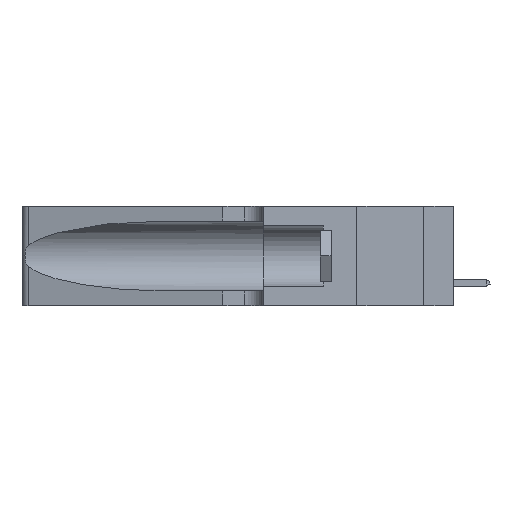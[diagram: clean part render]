
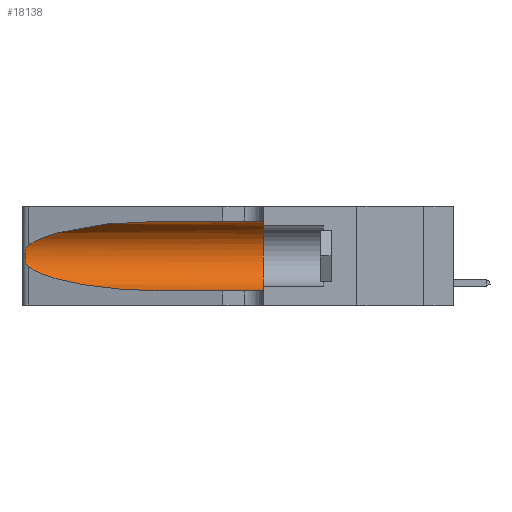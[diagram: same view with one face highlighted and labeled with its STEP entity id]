
A CAD part, left-side view. The second image highlights one B-rep face of the part: STEP entity #18138.
In plain terms, the highlighted cylindrical face has radius 3.308 mm (diameter 6.617 mm), a partial arc.
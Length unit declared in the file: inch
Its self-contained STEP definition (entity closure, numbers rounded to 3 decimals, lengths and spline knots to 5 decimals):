
#932 = CARTESIAN_POINT ( 'NONE',  ( 0.1305, 0.35, 0.185 ) ) ;
#1076 = CARTESIAN_POINT ( 'NONE',  ( 0.25856, 1.23593, 0.16098 ) ) ;
#1117 = CARTESIAN_POINT ( 'NONE',  ( 0.26017, 1.23833, 0.17102 ) ) ;
#2257 = CARTESIAN_POINT ( 'NONE',  ( 0.1305, 0.72297, 0.05475 ) ) ;
#2524 = CARTESIAN_POINT ( 'NONE',  ( 0.25555, 1.22993, 0.14849 ) ) ;
#4168 = CARTESIAN_POINT ( 'NONE',  ( 0.25487, 1.22718, 0.22369 ) ) ;
#4170 = CARTESIAN_POINT ( 'NONE',  ( 0.26018, 1.23835, 0.19895 ) ) ;
#4214 = VERTEX_POINT ( 'NONE', #36237 ) ;
#4315 = AXIS2_PLACEMENT_3D ( 'NONE', #32314, #23668, #15183 ) ;
#5307 = CARTESIAN_POINT ( 'NONE',  ( 0.25639, 1.23186, 0.15144 ) ) ;
#5326 = CARTESIAN_POINT ( 'NONE',  ( 0.25487, 1.22718, 0.14631 ) ) ;
#5389 = VERTEX_POINT ( 'NONE', #35864 ) ;
#5390 = LINE ( 'NONE', #26961, #9056 ) ;
#6180 = CARTESIAN_POINT ( 'NONE',  ( 0.25854, 1.2359, 0.20912 ) ) ;
#6542 = CARTESIAN_POINT ( 'NONE',  ( 0.2373, 1.15595, 0.28018 ) ) ;
#7054 = CARTESIAN_POINT ( 'NONE',  ( 0.26075, 1.23896, 0.19203 ) ) ;
#8023 = FACE_OUTER_BOUND ( 'NONE', #11184, .T. ) ;
#8202 = CARTESIAN_POINT ( 'NONE',  ( 0.25487, 1.22718, 0.22369 ) ) ;
#8237 =( BOUNDED_CURVE ( )  B_SPLINE_CURVE ( 3, ( #5326, #20031, #20159, #31861 ),
 .UNSPECIFIED., .F., .F. ) 
 B_SPLINE_CURVE_WITH_KNOTS ( ( 4, 4 ),
 ( 3.44316, 4.71239 ),
 .UNSPECIFIED. ) 
 CURVE ( )  GEOMETRIC_REPRESENTATION_ITEM ( )  RATIONAL_B_SPLINE_CURVE ( ( 1., 0.87, 0.87, 1. ) ) 
 REPRESENTATION_ITEM ( '' )  );
#8505 = CARTESIAN_POINT ( 'NONE',  ( 0.25787, 1.23484, 0.2124 ) ) ;
#8690 = VERTEX_POINT ( 'NONE', #2257 ) ;
#9056 = VECTOR ( 'NONE', #27078, 39.37008 ) ;
#9709 = DIRECTION ( 'NONE',  ( 0., 0., 1. ) ) ;
#11184 = EDGE_LOOP ( 'NONE', ( #12846, #19940, #32505, #31357, #23816, #23075 ) ) ;
#11272 = CARTESIAN_POINT ( 'NONE',  ( 0.25555, 1.22994, 0.2215 ) ) ;
#11501 = VERTEX_POINT ( 'NONE', #32273 ) ;
#12846 = ORIENTED_EDGE ( 'NONE', *, *, #26198, .T. ) ;
#13115 = CIRCLE ( 'NONE', #24609, 0.13025 ) ;
#13120 = EDGE_CURVE ( 'NONE', #4214, #14549, #22203, .T. ) ;
#13679 = CARTESIAN_POINT ( 'NONE',  ( 0.1305, 1.61858, 0.05475 ) ) ;
#14549 = VERTEX_POINT ( 'NONE', #37258 ) ;
#15183 = DIRECTION ( 'NONE',  ( 0., 0., -1. ) ) ;
#15453 = CARTESIAN_POINT ( 'NONE',  ( 0.1305, 0.72297, 0.31525 ) ) ;
#16664 = CYLINDRICAL_SURFACE ( 'NONE', #4315, 0.13025 ) ;
#17375 = VECTOR ( 'NONE', #36932, 39.37008 ) ;
#18138 = ADVANCED_FACE ( 'NONE', ( #8023 ), #16664, .F. ) ;
#19478 = CARTESIAN_POINT ( 'NONE',  ( 0.25789, 1.23486, 0.15765 ) ) ;
#19940 = ORIENTED_EDGE ( 'NONE', *, *, #13120, .T. ) ;
#20031 = CARTESIAN_POINT ( 'NONE',  ( 0.2373, 1.15595, 0.08982 ) ) ;
#20159 = CARTESIAN_POINT ( 'NONE',  ( 0.18966, 0.96281, 0.05475 ) ) ;
#20224 = CARTESIAN_POINT ( 'NONE',  ( 0.26075, 1.23896, 0.178 ) ) ;
#20244 = CARTESIAN_POINT ( 'NONE',  ( 0.25487, 1.22718, 0.14631 ) ) ;
#20422 = EDGE_CURVE ( 'NONE', #8690, #11501, #28761, .T. ) ;
#21249 = DIRECTION ( 'NONE',  ( 0., 1., 0. ) ) ;
#22203 = B_SPLINE_CURVE_WITH_KNOTS ( 'NONE', 3,
 ( #8202, #11272, #32216, #8505, #6180, #4170, #7054, #20224, #1117, #1076, #19478, #5307, #2524, #20244 ),
 .UNSPECIFIED., .F., .F.,
 ( 4, 2, 2, 2, 2, 2, 4 ),
 ( 0., 0.00027, 0.00053, 0.00107, 0.0016, 0.00187, 0.00214 ),
 .UNSPECIFIED. ) ;
#22978 = EDGE_CURVE ( 'NONE', #34588, #5389, #5390, .T. ) ;
#22985 = EDGE_CURVE ( 'NONE', #5389, #11501, #13115, .T. ) ;
#23075 = ORIENTED_EDGE ( 'NONE', *, *, #22978, .F. ) ;
#23668 = DIRECTION ( 'NONE',  ( 0., -1., 0. ) ) ;
#23816 = ORIENTED_EDGE ( 'NONE', *, *, #22985, .F. ) ;
#24609 = AXIS2_PLACEMENT_3D ( 'NONE', #932, #21249, #9709 ) ;
#25981 = EDGE_CURVE ( 'NONE', #14549, #8690, #8237, .T. ) ;
#26198 = EDGE_CURVE ( 'NONE', #34588, #4214, #29182, .T. ) ;
#26961 = CARTESIAN_POINT ( 'NONE',  ( 0.1305, 1.61858, 0.31525 ) ) ;
#27078 = DIRECTION ( 'NONE',  ( 0., -1., 0. ) ) ;
#27109 = CARTESIAN_POINT ( 'NONE',  ( 0.18966, 0.96281, 0.31525 ) ) ;
#28761 = LINE ( 'NONE', #13679, #17375 ) ;
#29182 =( BOUNDED_CURVE ( )  B_SPLINE_CURVE ( 3, ( #15453, #27109, #6542, #4168 ),
 .UNSPECIFIED., .F., .T. ) 
 B_SPLINE_CURVE_WITH_KNOTS ( ( 4, 4 ),
 ( 1.5708, 2.84003 ),
 .UNSPECIFIED. ) 
 CURVE ( )  GEOMETRIC_REPRESENTATION_ITEM ( )  RATIONAL_B_SPLINE_CURVE ( ( 1., 0.87, 0.87, 1. ) ) 
 REPRESENTATION_ITEM ( '' )  );
#31357 = ORIENTED_EDGE ( 'NONE', *, *, #20422, .T. ) ;
#31861 = CARTESIAN_POINT ( 'NONE',  ( 0.1305, 0.72297, 0.05475 ) ) ;
#32216 = CARTESIAN_POINT ( 'NONE',  ( 0.25639, 1.23184, 0.21858 ) ) ;
#32273 = CARTESIAN_POINT ( 'NONE',  ( 0.1305, 0.35, 0.05475 ) ) ;
#32314 = CARTESIAN_POINT ( 'NONE',  ( 0.1305, 1.61858, 0.185 ) ) ;
#32505 = ORIENTED_EDGE ( 'NONE', *, *, #25981, .T. ) ;
#32759 = CARTESIAN_POINT ( 'NONE',  ( 0.1305, 0.72297, 0.31525 ) ) ;
#34588 = VERTEX_POINT ( 'NONE', #32759 ) ;
#35864 = CARTESIAN_POINT ( 'NONE',  ( 0.1305, 0.35, 0.31525 ) ) ;
#36237 = CARTESIAN_POINT ( 'NONE',  ( 0.25487, 1.22718, 0.22369 ) ) ;
#36932 = DIRECTION ( 'NONE',  ( 0., -1., 0. ) ) ;
#37258 = CARTESIAN_POINT ( 'NONE',  ( 0.25487, 1.22718, 0.14631 ) ) ;
